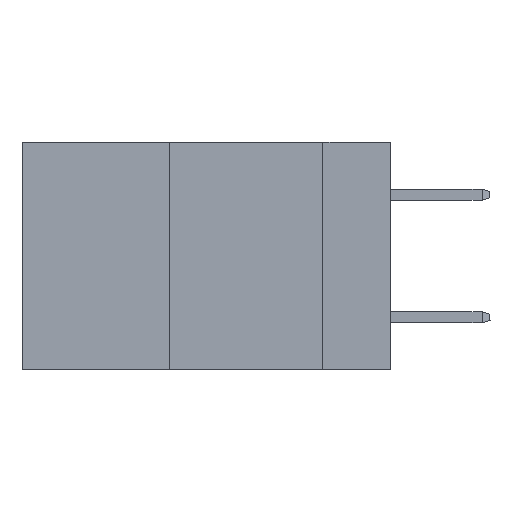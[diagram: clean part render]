
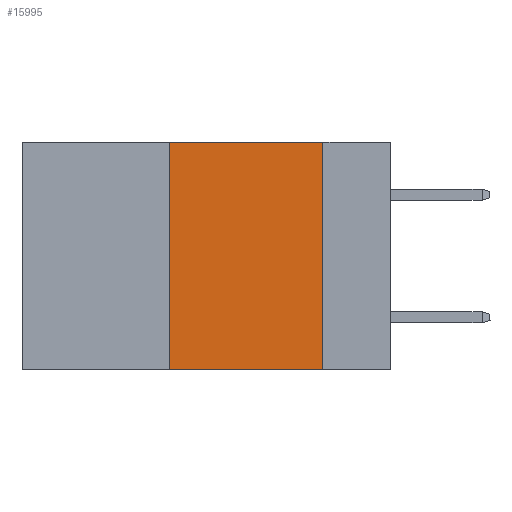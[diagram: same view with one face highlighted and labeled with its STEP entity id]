
A CAD part, left-side view. The second image highlights one B-rep face of the part: STEP entity #15995.
In plain terms, the highlighted planar face has unit normal (-1, 0, 0).
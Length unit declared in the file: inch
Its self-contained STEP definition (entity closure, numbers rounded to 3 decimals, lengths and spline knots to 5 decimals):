
#224 = LINE ( 'NONE', #6544, #15180 ) ;
#800 = EDGE_LOOP ( 'NONE', ( #21279, #25281, #6792, #15103 ) ) ;
#1076 = VECTOR ( 'NONE', #4122, 39.37008 ) ;
#3637 = EDGE_CURVE ( 'NONE', #25214, #5206, #6219, .T. ) ;
#4122 = DIRECTION ( 'NONE',  ( 0., 0., -1. ) ) ;
#4134 = EDGE_CURVE ( 'NONE', #16990, #25214, #23926, .T. ) ;
#4615 = CARTESIAN_POINT ( 'NONE',  ( 0., 0.6, 0. ) ) ;
#5206 = VERTEX_POINT ( 'NONE', #9068 ) ;
#5613 = DIRECTION ( 'NONE',  ( 0., -1., 0. ) ) ;
#6219 = LINE ( 'NONE', #17235, #1076 ) ;
#6349 = CARTESIAN_POINT ( 'NONE',  ( 0., 0.11, 0. ) ) ;
#6544 = CARTESIAN_POINT ( 'NONE',  ( 0., 0.6, -0.37 ) ) ;
#6792 = ORIENTED_EDGE ( 'NONE', *, *, #9650, .F. ) ;
#8798 = DIRECTION ( 'NONE',  ( 0., 0., -1. ) ) ;
#9068 = CARTESIAN_POINT ( 'NONE',  ( 0., 0.11, -0.37 ) ) ;
#9650 = EDGE_CURVE ( 'NONE', #18698, #16990, #14456, .T. ) ;
#10619 = DIRECTION ( 'NONE',  ( 0., 0., 1. ) ) ;
#11182 = CARTESIAN_POINT ( 'NONE',  ( 0., 0.6, 0. ) ) ;
#12094 = FACE_OUTER_BOUND ( 'NONE', #800, .T. ) ;
#12574 = AXIS2_PLACEMENT_3D ( 'NONE', #4615, #20581, #8798 ) ;
#12646 = PLANE ( 'NONE',  #12574 ) ;
#14381 = CARTESIAN_POINT ( 'NONE',  ( 0., 0.36, 0. ) ) ;
#14456 = LINE ( 'NONE', #14381, #15683 ) ;
#14514 = CARTESIAN_POINT ( 'NONE',  ( 0., 0.36, -0.37 ) ) ;
#15103 = ORIENTED_EDGE ( 'NONE', *, *, #16831, .T. ) ;
#15180 = VECTOR ( 'NONE', #18376, 39.37008 ) ;
#15683 = VECTOR ( 'NONE', #10619, 39.37008 ) ;
#15995 = ADVANCED_FACE ( 'NONE', ( #12094 ), #12646, .F. ) ;
#16831 = EDGE_CURVE ( 'NONE', #18698, #5206, #224, .T. ) ;
#16990 = VERTEX_POINT ( 'NONE', #18810 ) ;
#17235 = CARTESIAN_POINT ( 'NONE',  ( 0., 0.11, 0. ) ) ;
#18376 = DIRECTION ( 'NONE',  ( 0., -1., 0. ) ) ;
#18401 = VECTOR ( 'NONE', #5613, 39.37008 ) ;
#18698 = VERTEX_POINT ( 'NONE', #14514 ) ;
#18810 = CARTESIAN_POINT ( 'NONE',  ( 0., 0.36, 0. ) ) ;
#20581 = DIRECTION ( 'NONE',  ( 1., 0., 0. ) ) ;
#21279 = ORIENTED_EDGE ( 'NONE', *, *, #3637, .F. ) ;
#23926 = LINE ( 'NONE', #11182, #18401 ) ;
#25214 = VERTEX_POINT ( 'NONE', #6349 ) ;
#25281 = ORIENTED_EDGE ( 'NONE', *, *, #4134, .F. ) ;
